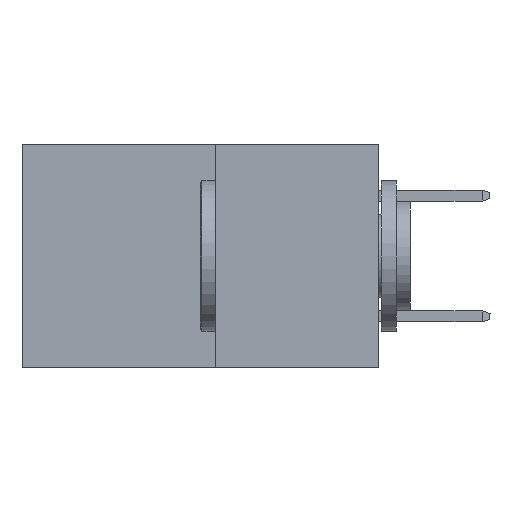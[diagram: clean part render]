
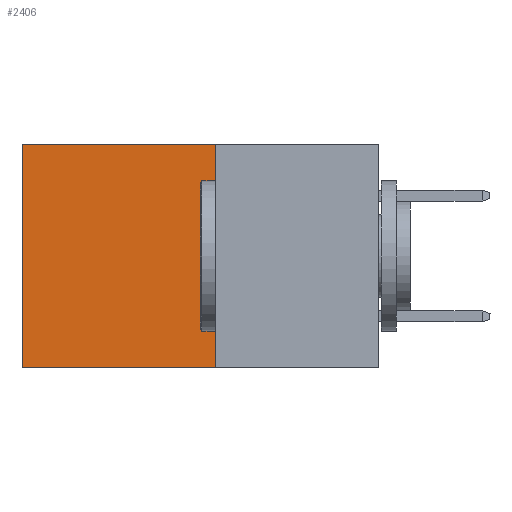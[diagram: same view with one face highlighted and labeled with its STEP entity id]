
A CAD part, left-side view. The second image highlights one B-rep face of the part: STEP entity #2406.
In plain terms, the highlighted planar face has unit normal (-1, 0, 0).
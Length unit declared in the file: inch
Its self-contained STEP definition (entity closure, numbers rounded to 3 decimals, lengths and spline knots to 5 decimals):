
#618 = LINE ( 'NONE', #23793, #6217 ) ;
#628 = VERTEX_POINT ( 'NONE', #24830 ) ;
#1408 = EDGE_CURVE ( 'NONE', #16822, #628, #23421, .T. ) ;
#2101 = CARTESIAN_POINT ( 'NONE',  ( 0.277, 0.59, -0.37 ) ) ;
#2256 = CARTESIAN_POINT ( 'NONE',  ( 0.277, 0.59, 0. ) ) ;
#2406 = ADVANCED_FACE ( 'NONE', ( #6873 ), #16346, .F. ) ;
#2879 = VERTEX_POINT ( 'NONE', #2256 ) ;
#4933 = VECTOR ( 'NONE', #13069, 39.37008 ) ;
#6217 = VECTOR ( 'NONE', #26440, 39.37008 ) ;
#6873 = FACE_OUTER_BOUND ( 'NONE', #25166, .T. ) ;
#7794 = LINE ( 'NONE', #10058, #15834 ) ;
#9287 = CARTESIAN_POINT ( 'NONE',  ( 0.277, 0.27, -0.37 ) ) ;
#10058 = CARTESIAN_POINT ( 'NONE',  ( 0.277, 0.27, -0.37 ) ) ;
#10244 = EDGE_CURVE ( 'NONE', #16822, #2879, #618, .T. ) ;
#10426 = CARTESIAN_POINT ( 'NONE',  ( 0.277, 0.27, 0. ) ) ;
#12134 = LINE ( 'NONE', #2101, #4933 ) ;
#13069 = DIRECTION ( 'NONE',  ( 0., 0., -1. ) ) ;
#14044 = ORIENTED_EDGE ( 'NONE', *, *, #18580, .F. ) ;
#14731 = DIRECTION ( 'NONE',  ( 0., 0., -1. ) ) ;
#15834 = VECTOR ( 'NONE', #31491, 39.37008 ) ;
#16196 = DIRECTION ( 'NONE',  ( 1., 0., 0. ) ) ;
#16346 = PLANE ( 'NONE',  #27518 ) ;
#16762 = ORIENTED_EDGE ( 'NONE', *, *, #25135, .T. ) ;
#16822 = VERTEX_POINT ( 'NONE', #10426 ) ;
#18580 = EDGE_CURVE ( 'NONE', #628, #26203, #7794, .T. ) ;
#22591 = VECTOR ( 'NONE', #31315, 39.37008 ) ;
#23421 = LINE ( 'NONE', #26384, #22591 ) ;
#23793 = CARTESIAN_POINT ( 'NONE',  ( 0.277, 0.27, 0. ) ) ;
#24830 = CARTESIAN_POINT ( 'NONE',  ( 0.277, 0.27, -0.37 ) ) ;
#25135 = EDGE_CURVE ( 'NONE', #2879, #26203, #12134, .T. ) ;
#25166 = EDGE_LOOP ( 'NONE', ( #16762, #14044, #25649, #31127 ) ) ;
#25649 = ORIENTED_EDGE ( 'NONE', *, *, #1408, .F. ) ;
#26203 = VERTEX_POINT ( 'NONE', #30901 ) ;
#26384 = CARTESIAN_POINT ( 'NONE',  ( 0.277, 0.27, -0.37 ) ) ;
#26440 = DIRECTION ( 'NONE',  ( 0., 1., 0. ) ) ;
#27518 = AXIS2_PLACEMENT_3D ( 'NONE', #9287, #16196, #14731 ) ;
#30901 = CARTESIAN_POINT ( 'NONE',  ( 0.277, 0.59, -0.37 ) ) ;
#31127 = ORIENTED_EDGE ( 'NONE', *, *, #10244, .T. ) ;
#31315 = DIRECTION ( 'NONE',  ( 0., 0., -1. ) ) ;
#31491 = DIRECTION ( 'NONE',  ( 0., 1., 0. ) ) ;
